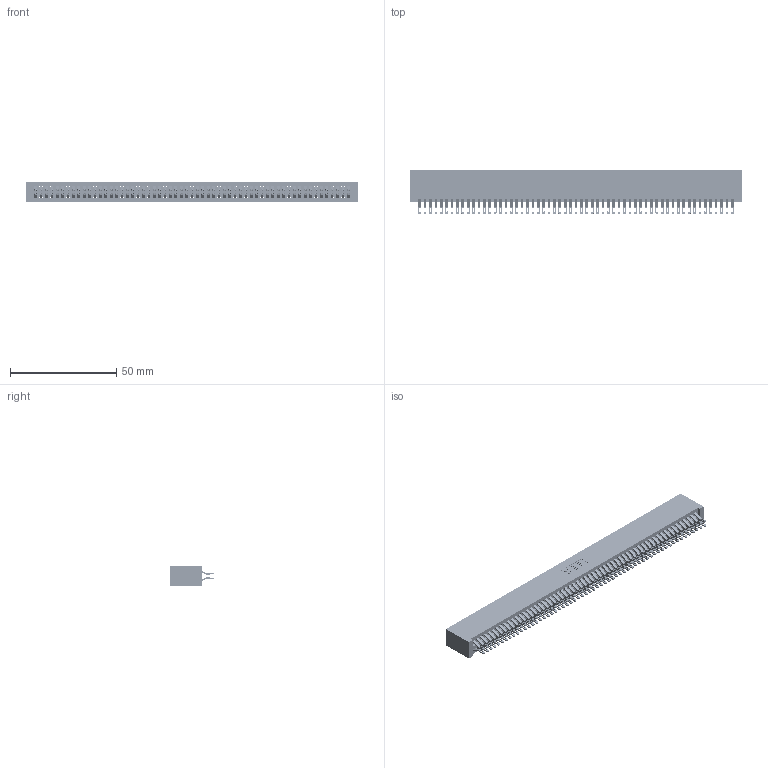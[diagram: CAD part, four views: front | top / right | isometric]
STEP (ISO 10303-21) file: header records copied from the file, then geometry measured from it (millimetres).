
FILE_DESCRIPTION (( 'STEP AP203' ), '1' );
FILE_NAME ('345-118-555-201.STEP', '2019-11-05T21:11:13', ( '' ), ( '' ), 'SwSTEP 2.0', 'SolidWorks 2016', '' );
FILE_SCHEMA (( 'CONFIG_CONTROL_DESIGN' ));
Length unit declared in the file: inch
Products named in the file (3): 345-118-555-201; 345 Part_No Mounting Lugs; 345-292-001_555 Tail
Assembly tree (119 placements, depth 2):
  345-118-555-201
    345 Part_No Mounting Lugs
    345-292-001_555 Tail  x118
Bounding box: 156.46 x 21.13 x 9.4 mm (x, y, z)
Volume: 16315 mm3; surface area: 25939.3 mm2
Topology: 119 solids, 119 shells, 6726 faces, 21203 edges, 14134 vertices
Faces by surface type: plane 3734, cylinder 2992
Entity records: 44053 total; most frequent: CARTESIAN_POINT 7402, ORIENTED_EDGE 7306, DIRECTION 6469, EDGE_CURVE 3653, VECTOR 3273, LINE 3273, VERTEX_POINT 2434, AXIS2_PLACEMENT_3D 1598
